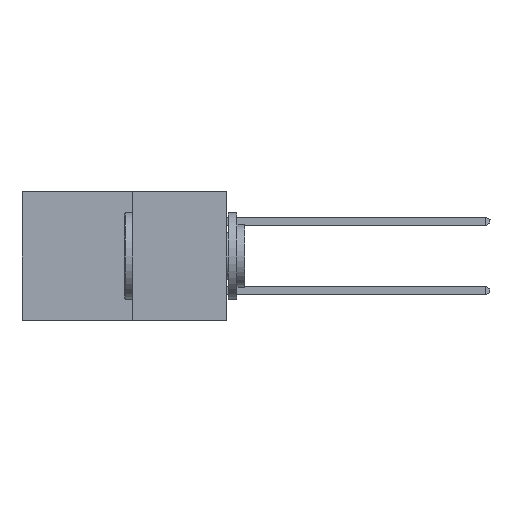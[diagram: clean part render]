
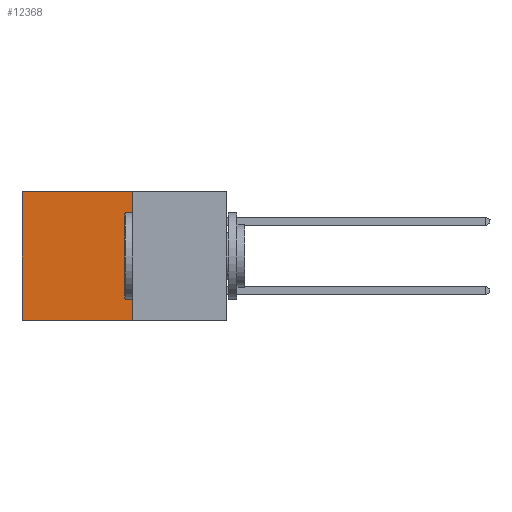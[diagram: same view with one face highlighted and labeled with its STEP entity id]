
A CAD part, left-side view. The second image highlights one B-rep face of the part: STEP entity #12368.
In plain terms, the highlighted planar face has unit normal (-1, 0, 0).
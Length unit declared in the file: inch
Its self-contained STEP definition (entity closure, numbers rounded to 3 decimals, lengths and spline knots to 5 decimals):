
#651 = CARTESIAN_POINT ( 'NONE',  ( 0.277, 0.59, -0.37 ) ) ;
#1341 = VERTEX_POINT ( 'NONE', #3554 ) ;
#3107 = LINE ( 'NONE', #12115, #16998 ) ;
#3154 = DIRECTION ( 'NONE',  ( 0., 0., -1. ) ) ;
#3554 = CARTESIAN_POINT ( 'NONE',  ( 0.277, 0.27, -0.37 ) ) ;
#4132 = LINE ( 'NONE', #16988, #10657 ) ;
#4766 = DIRECTION ( 'NONE',  ( 1., 0., 0. ) ) ;
#5756 = ORIENTED_EDGE ( 'NONE', *, *, #7707, .T. ) ;
#6123 = DIRECTION ( 'NONE',  ( 0., 1., 0. ) ) ;
#6215 = CARTESIAN_POINT ( 'NONE',  ( 0.277, 0.27, 0. ) ) ;
#6398 = ORIENTED_EDGE ( 'NONE', *, *, #17068, .F. ) ;
#7707 = EDGE_CURVE ( 'NONE', #18429, #31920, #30352, .T. ) ;
#8299 = VECTOR ( 'NONE', #6123, 39.37008 ) ;
#9456 = CARTESIAN_POINT ( 'NONE',  ( 0.277, 0.27, -0.37 ) ) ;
#10374 = ORIENTED_EDGE ( 'NONE', *, *, #28631, .F. ) ;
#10657 = VECTOR ( 'NONE', #3154, 39.37008 ) ;
#12115 = CARTESIAN_POINT ( 'NONE',  ( 0.277, 0.59, -0.37 ) ) ;
#12368 = ADVANCED_FACE ( 'NONE', ( #17440 ), #35067, .F. ) ;
#14882 = DIRECTION ( 'NONE',  ( 0., 0., -1. ) ) ;
#14971 = DIRECTION ( 'NONE',  ( 0., 1., 0. ) ) ;
#15917 = VERTEX_POINT ( 'NONE', #651 ) ;
#16988 = CARTESIAN_POINT ( 'NONE',  ( 0.277, 0.27, -0.37 ) ) ;
#16998 = VECTOR ( 'NONE', #14882, 39.37008 ) ;
#17068 = EDGE_CURVE ( 'NONE', #18429, #1341, #4132, .T. ) ;
#17440 = FACE_OUTER_BOUND ( 'NONE', #28393, .T. ) ;
#18429 = VERTEX_POINT ( 'NONE', #32084 ) ;
#18603 = CARTESIAN_POINT ( 'NONE',  ( 0.277, 0.27, -0.37 ) ) ;
#21113 = ORIENTED_EDGE ( 'NONE', *, *, #30012, .T. ) ;
#24149 = AXIS2_PLACEMENT_3D ( 'NONE', #18603, #4766, #24165 ) ;
#24165 = DIRECTION ( 'NONE',  ( 0., 0., -1. ) ) ;
#24483 = LINE ( 'NONE', #9456, #31788 ) ;
#26858 = CARTESIAN_POINT ( 'NONE',  ( 0.277, 0.59, 0. ) ) ;
#28393 = EDGE_LOOP ( 'NONE', ( #21113, #10374, #6398, #5756 ) ) ;
#28631 = EDGE_CURVE ( 'NONE', #1341, #15917, #24483, .T. ) ;
#30012 = EDGE_CURVE ( 'NONE', #31920, #15917, #3107, .T. ) ;
#30352 = LINE ( 'NONE', #6215, #8299 ) ;
#31788 = VECTOR ( 'NONE', #14971, 39.37008 ) ;
#31920 = VERTEX_POINT ( 'NONE', #26858 ) ;
#32084 = CARTESIAN_POINT ( 'NONE',  ( 0.277, 0.27, 0. ) ) ;
#35067 = PLANE ( 'NONE',  #24149 ) ;
